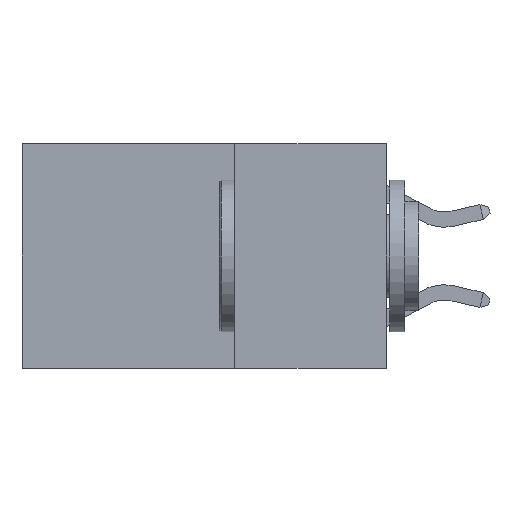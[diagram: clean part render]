
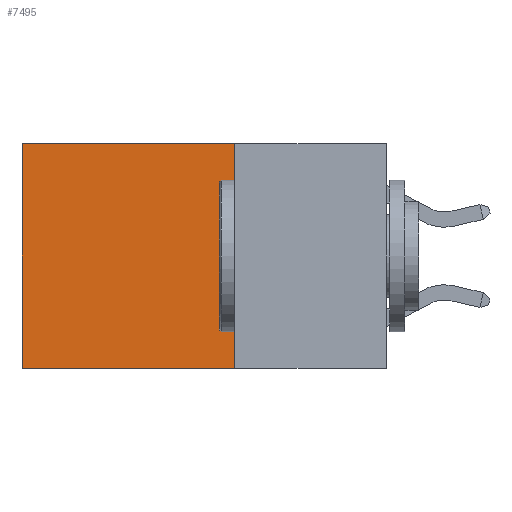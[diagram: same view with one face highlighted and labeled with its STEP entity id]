
A CAD part, left-side view. The second image highlights one B-rep face of the part: STEP entity #7495.
In plain terms, the highlighted planar face has unit normal (-1, 0, 0).
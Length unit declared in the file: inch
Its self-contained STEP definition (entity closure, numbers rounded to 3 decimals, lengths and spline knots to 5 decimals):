
#356 = LINE ( 'NONE', #10756, #9501 ) ;
#1008 = AXIS2_PLACEMENT_3D ( 'NONE', #5380, #2723, #8941 ) ;
#1062 = EDGE_CURVE ( 'NONE', #2946, #10828, #11022, .T. ) ;
#1788 = VERTEX_POINT ( 'NONE', #9457 ) ;
#2100 = EDGE_CURVE ( 'NONE', #1788, #4215, #2236, .T. ) ;
#2126 = VECTOR ( 'NONE', #5899, 39.37008 ) ;
#2236 = LINE ( 'NONE', #6445, #6683 ) ;
#2702 = DIRECTION ( 'NONE',  ( 0., 1., 0. ) ) ;
#2723 = DIRECTION ( 'NONE',  ( 1., 0., 0. ) ) ;
#2888 = ORIENTED_EDGE ( 'NONE', *, *, #1062, .T. ) ;
#2931 = ORIENTED_EDGE ( 'NONE', *, *, #3235, .F. ) ;
#2946 = VERTEX_POINT ( 'NONE', #4389 ) ;
#2965 = ORIENTED_EDGE ( 'NONE', *, *, #2100, .F. ) ;
#3235 = EDGE_CURVE ( 'NONE', #4215, #10828, #4932, .T. ) ;
#3576 = ORIENTED_EDGE ( 'NONE', *, *, #8584, .T. ) ;
#4215 = VERTEX_POINT ( 'NONE', #8527 ) ;
#4296 = CARTESIAN_POINT ( 'NONE',  ( 0.2625, 0.6, -0.37 ) ) ;
#4389 = CARTESIAN_POINT ( 'NONE',  ( 0.2625, 0.6, 0. ) ) ;
#4793 = DIRECTION ( 'NONE',  ( 0., 1., 0. ) ) ;
#4932 = LINE ( 'NONE', #5586, #7022 ) ;
#5380 = CARTESIAN_POINT ( 'NONE',  ( 0.2625, 0.25, 0. ) ) ;
#5586 = CARTESIAN_POINT ( 'NONE',  ( 0.2625, 0.25, -0.37 ) ) ;
#5899 = DIRECTION ( 'NONE',  ( 0., 0., -1. ) ) ;
#5955 = CARTESIAN_POINT ( 'NONE',  ( 0.2625, 0.6, 0. ) ) ;
#6403 = DIRECTION ( 'NONE',  ( 0., 0., -1. ) ) ;
#6445 = CARTESIAN_POINT ( 'NONE',  ( 0.2625, 0.25, 0. ) ) ;
#6683 = VECTOR ( 'NONE', #6403, 39.37008 ) ;
#7022 = VECTOR ( 'NONE', #2702, 39.37008 ) ;
#7495 = ADVANCED_FACE ( 'NONE', ( #7862 ), #8024, .F. ) ;
#7862 = FACE_OUTER_BOUND ( 'NONE', #9531, .T. ) ;
#8024 = PLANE ( 'NONE',  #1008 ) ;
#8527 = CARTESIAN_POINT ( 'NONE',  ( 0.2625, 0.25, -0.37 ) ) ;
#8584 = EDGE_CURVE ( 'NONE', #1788, #2946, #356, .T. ) ;
#8941 = DIRECTION ( 'NONE',  ( 0., 0., -1. ) ) ;
#9457 = CARTESIAN_POINT ( 'NONE',  ( 0.2625, 0.25, 0. ) ) ;
#9501 = VECTOR ( 'NONE', #4793, 39.37008 ) ;
#9531 = EDGE_LOOP ( 'NONE', ( #2888, #2931, #2965, #3576 ) ) ;
#10756 = CARTESIAN_POINT ( 'NONE',  ( 0.2625, 0.25, 0. ) ) ;
#10828 = VERTEX_POINT ( 'NONE', #4296 ) ;
#11022 = LINE ( 'NONE', #5955, #2126 ) ;
